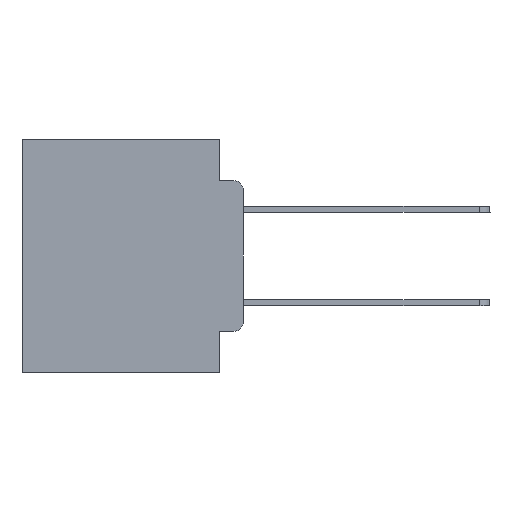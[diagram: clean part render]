
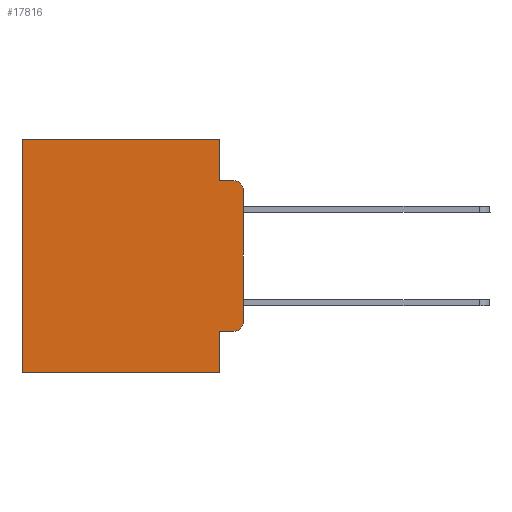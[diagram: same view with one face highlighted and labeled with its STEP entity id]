
A CAD part, left-side view. The second image highlights one B-rep face of the part: STEP entity #17816.
In plain terms, the highlighted planar face has unit normal (-1, 0, 0).
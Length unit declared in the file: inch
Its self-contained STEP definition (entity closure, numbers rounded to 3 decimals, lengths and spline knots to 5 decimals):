
#255 = VERTEX_POINT ( 'NONE', #21651 ) ;
#395 = DIRECTION ( 'NONE',  ( 1., 0., 0. ) ) ;
#774 = CARTESIAN_POINT ( 'NONE',  ( 0.298, 0.051, -0.0885 ) ) ;
#849 = PLANE ( 'NONE',  #27355 ) ;
#1015 = DIRECTION ( 'NONE',  ( 0., 0., -1. ) ) ;
#1174 = ORIENTED_EDGE ( 'NONE', *, *, #18419, .T. ) ;
#1544 = CARTESIAN_POINT ( 'NONE',  ( 0.298, 0., -0.5 ) ) ;
#1794 = VERTEX_POINT ( 'NONE', #774 ) ;
#2122 = VERTEX_POINT ( 'NONE', #20119 ) ;
#2502 = CARTESIAN_POINT ( 'NONE',  ( 0.298, 0.051, 0. ) ) ;
#2559 = VERTEX_POINT ( 'NONE', #19654 ) ;
#2646 = AXIS2_PLACEMENT_3D ( 'NONE', #3979, #6636, #26597 ) ;
#3750 = DIRECTION ( 'NONE',  ( 0., 0., -1. ) ) ;
#3979 = CARTESIAN_POINT ( 'NONE',  ( 0.298, 0.02, -0.1085 ) ) ;
#4895 = CARTESIAN_POINT ( 'NONE',  ( 0.298, 0.473, -0.5 ) ) ;
#5266 = ORIENTED_EDGE ( 'NONE', *, *, #25418, .T. ) ;
#5644 = VECTOR ( 'NONE', #12653, 39.37008 ) ;
#5770 = LINE ( 'NONE', #21110, #18656 ) ;
#6230 = ORIENTED_EDGE ( 'NONE', *, *, #23715, .T. ) ;
#6374 = FACE_OUTER_BOUND ( 'NONE', #6542, .T. ) ;
#6509 = CARTESIAN_POINT ( 'NONE',  ( 0.298, 0.02, -0.3915 ) ) ;
#6542 = EDGE_LOOP ( 'NONE', ( #6774, #6230, #20932, #9408, #1174, #27122, #26470, #26903, #28829, #5266 ) ) ;
#6636 = DIRECTION ( 'NONE',  ( -1., 0., 0. ) ) ;
#6774 = ORIENTED_EDGE ( 'NONE', *, *, #27980, .F. ) ;
#7066 = CARTESIAN_POINT ( 'NONE',  ( 0.298, 0., 0. ) ) ;
#7458 = VERTEX_POINT ( 'NONE', #4895 ) ;
#7548 = VERTEX_POINT ( 'NONE', #29307 ) ;
#8467 = DIRECTION ( 'NONE',  ( 0., -1., 0. ) ) ;
#8519 = EDGE_CURVE ( 'NONE', #24899, #2559, #29001, .T. ) ;
#9042 = DIRECTION ( 'NONE',  ( 0., 0., -1. ) ) ;
#9389 = AXIS2_PLACEMENT_3D ( 'NONE', #6509, #20498, #9042 ) ;
#9408 = ORIENTED_EDGE ( 'NONE', *, *, #28399, .F. ) ;
#9637 = LINE ( 'NONE', #25560, #14766 ) ;
#10225 = EDGE_CURVE ( 'NONE', #24899, #13046, #5770, .T. ) ;
#11624 = VECTOR ( 'NONE', #17488, 39.37008 ) ;
#11694 = DIRECTION ( 'NONE',  ( 0., 1., 0. ) ) ;
#11743 = CARTESIAN_POINT ( 'NONE',  ( 0.298, 0., -0.3915 ) ) ;
#12249 = LINE ( 'NONE', #28607, #18962 ) ;
#12653 = DIRECTION ( 'NONE',  ( 0., 0., -1. ) ) ;
#12723 = LINE ( 'NONE', #1544, #11624 ) ;
#13046 = VERTEX_POINT ( 'NONE', #22365 ) ;
#14240 = CARTESIAN_POINT ( 'NONE',  ( 0.298, 0.473, 0. ) ) ;
#14252 = EDGE_CURVE ( 'NONE', #13046, #7458, #12723, .T. ) ;
#14766 = VECTOR ( 'NONE', #25121, 39.37008 ) ;
#15056 = VECTOR ( 'NONE', #11694, 39.37008 ) ;
#15496 = CIRCLE ( 'NONE', #2646, 0.02 ) ;
#16348 = CARTESIAN_POINT ( 'NONE',  ( 0.298, 0., 0. ) ) ;
#16648 = DIRECTION ( 'NONE',  ( 0., 0., -1. ) ) ;
#17254 = CARTESIAN_POINT ( 'NONE',  ( 0.298, 0.051, -0.4115 ) ) ;
#17488 = DIRECTION ( 'NONE',  ( 0., 1., 0. ) ) ;
#17816 = ADVANCED_FACE ( 'NONE', ( #6374 ), #849, .F. ) ;
#18419 = EDGE_CURVE ( 'NONE', #28700, #255, #27452, .T. ) ;
#18455 = VECTOR ( 'NONE', #8467, 39.37008 ) ;
#18656 = VECTOR ( 'NONE', #1015, 39.37008 ) ;
#18962 = VECTOR ( 'NONE', #3750, 39.37008 ) ;
#19208 = CARTESIAN_POINT ( 'NONE',  ( 0.298, 0.051, 0. ) ) ;
#19654 = CARTESIAN_POINT ( 'NONE',  ( 0.298, 0.02, -0.4115 ) ) ;
#19694 = EDGE_CURVE ( 'NONE', #255, #7458, #25530, .T. ) ;
#20119 = CARTESIAN_POINT ( 'NONE',  ( 0.298, 0., -0.1085 ) ) ;
#20306 = CIRCLE ( 'NONE', #9389, 0.02 ) ;
#20498 = DIRECTION ( 'NONE',  ( -1., 0., 0. ) ) ;
#20932 = ORIENTED_EDGE ( 'NONE', *, *, #21899, .F. ) ;
#21110 = CARTESIAN_POINT ( 'NONE',  ( 0.298, 0.051, 0. ) ) ;
#21303 = LINE ( 'NONE', #19208, #5644 ) ;
#21651 = CARTESIAN_POINT ( 'NONE',  ( 0.298, 0.473, 0. ) ) ;
#21899 = EDGE_CURVE ( 'NONE', #1794, #7548, #9637, .T. ) ;
#22365 = CARTESIAN_POINT ( 'NONE',  ( 0.298, 0.051, -0.5 ) ) ;
#23299 = DIRECTION ( 'NONE',  ( 0., 0., -1. ) ) ;
#23715 = EDGE_CURVE ( 'NONE', #2122, #7548, #15496, .T. ) ;
#24668 = VERTEX_POINT ( 'NONE', #11743 ) ;
#24899 = VERTEX_POINT ( 'NONE', #17254 ) ;
#25121 = DIRECTION ( 'NONE',  ( 0., -1., 0. ) ) ;
#25418 = EDGE_CURVE ( 'NONE', #2559, #24668, #20306, .T. ) ;
#25530 = LINE ( 'NONE', #14240, #27446 ) ;
#25560 = CARTESIAN_POINT ( 'NONE',  ( 0.298, 0.051, -0.0885 ) ) ;
#26470 = ORIENTED_EDGE ( 'NONE', *, *, #14252, .F. ) ;
#26478 = CARTESIAN_POINT ( 'NONE',  ( 0.298, 0.051, -0.4115 ) ) ;
#26597 = DIRECTION ( 'NONE',  ( 0., 0., -1. ) ) ;
#26903 = ORIENTED_EDGE ( 'NONE', *, *, #10225, .F. ) ;
#27122 = ORIENTED_EDGE ( 'NONE', *, *, #19694, .T. ) ;
#27355 = AXIS2_PLACEMENT_3D ( 'NONE', #16348, #395, #16648 ) ;
#27446 = VECTOR ( 'NONE', #23299, 39.37008 ) ;
#27452 = LINE ( 'NONE', #7066, #15056 ) ;
#27980 = EDGE_CURVE ( 'NONE', #2122, #24668, #12249, .T. ) ;
#28399 = EDGE_CURVE ( 'NONE', #28700, #1794, #21303, .T. ) ;
#28607 = CARTESIAN_POINT ( 'NONE',  ( 0.298, 0., 0. ) ) ;
#28700 = VERTEX_POINT ( 'NONE', #2502 ) ;
#28829 = ORIENTED_EDGE ( 'NONE', *, *, #8519, .T. ) ;
#29001 = LINE ( 'NONE', #26478, #18455 ) ;
#29307 = CARTESIAN_POINT ( 'NONE',  ( 0.298, 0.02, -0.0885 ) ) ;
